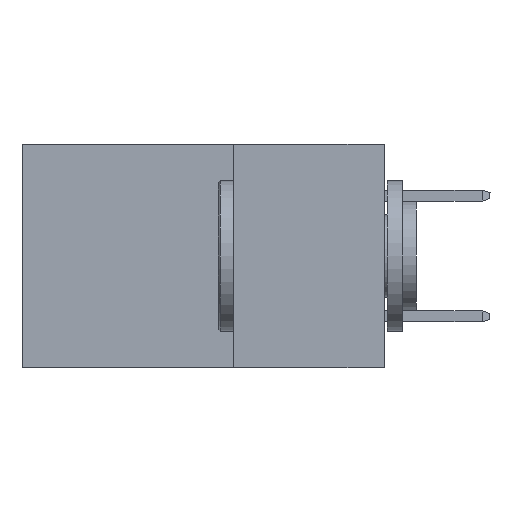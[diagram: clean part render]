
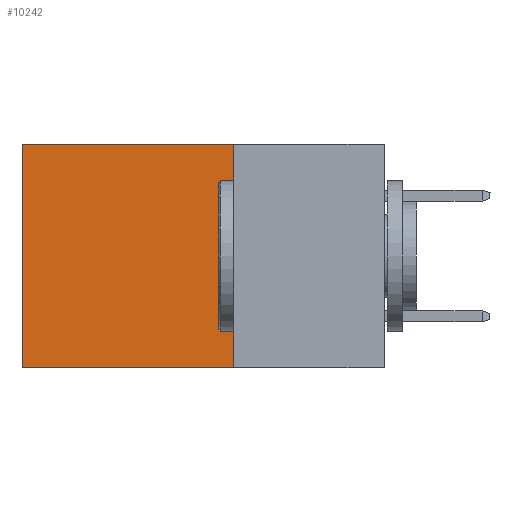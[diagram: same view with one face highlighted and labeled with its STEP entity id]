
A CAD part, left-side view. The second image highlights one B-rep face of the part: STEP entity #10242.
In plain terms, the highlighted planar face has unit normal (-1, 0, 0).
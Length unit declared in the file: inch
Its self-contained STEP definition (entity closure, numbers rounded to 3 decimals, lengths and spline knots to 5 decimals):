
#322 = ORIENTED_EDGE ( 'NONE', *, *, #11833, .F. ) ;
#599 = PLANE ( 'NONE',  #3656 ) ;
#931 = FACE_OUTER_BOUND ( 'NONE', #4082, .T. ) ;
#969 = VECTOR ( 'NONE', #11041, 39.37008 ) ;
#1170 = LINE ( 'NONE', #14396, #7731 ) ;
#1259 = DIRECTION ( 'NONE',  ( 0., 0., -1. ) ) ;
#1739 = LINE ( 'NONE', #15676, #4783 ) ;
#1925 = DIRECTION ( 'NONE',  ( 1., 0., 0. ) ) ;
#2004 = CARTESIAN_POINT ( 'NONE',  ( 0.298, 0.25, -0.37 ) ) ;
#3013 = LINE ( 'NONE', #5563, #969 ) ;
#3249 = DIRECTION ( 'NONE',  ( 0., 0., -1. ) ) ;
#3656 = AXIS2_PLACEMENT_3D ( 'NONE', #16466, #1925, #3249 ) ;
#4034 = CARTESIAN_POINT ( 'NONE',  ( 0.298, 0.25, 0. ) ) ;
#4082 = EDGE_LOOP ( 'NONE', ( #4154, #11042, #322, #10776 ) ) ;
#4154 = ORIENTED_EDGE ( 'NONE', *, *, #12080, .T. ) ;
#4472 = EDGE_CURVE ( 'NONE', #7704, #12834, #1739, .T. ) ;
#4566 = VECTOR ( 'NONE', #14187, 39.37008 ) ;
#4781 = CARTESIAN_POINT ( 'NONE',  ( 0.298, 0.25, -0.37 ) ) ;
#4783 = VECTOR ( 'NONE', #7977, 39.37008 ) ;
#5176 = EDGE_CURVE ( 'NONE', #15212, #11227, #9521, .T. ) ;
#5563 = CARTESIAN_POINT ( 'NONE',  ( 0.298, 0.6, 0. ) ) ;
#7704 = VERTEX_POINT ( 'NONE', #4034 ) ;
#7731 = VECTOR ( 'NONE', #1259, 39.37008 ) ;
#7977 = DIRECTION ( 'NONE',  ( 0., 1., 0. ) ) ;
#9449 = CARTESIAN_POINT ( 'NONE',  ( 0.298, 0.6, -0.37 ) ) ;
#9521 = LINE ( 'NONE', #4781, #4566 ) ;
#10242 = ADVANCED_FACE ( 'NONE', ( #931 ), #599, .F. ) ;
#10776 = ORIENTED_EDGE ( 'NONE', *, *, #4472, .T. ) ;
#11041 = DIRECTION ( 'NONE',  ( 0., 0., -1. ) ) ;
#11042 = ORIENTED_EDGE ( 'NONE', *, *, #5176, .F. ) ;
#11227 = VERTEX_POINT ( 'NONE', #9449 ) ;
#11833 = EDGE_CURVE ( 'NONE', #7704, #15212, #1170, .T. ) ;
#12080 = EDGE_CURVE ( 'NONE', #12834, #11227, #3013, .T. ) ;
#12834 = VERTEX_POINT ( 'NONE', #16276 ) ;
#14187 = DIRECTION ( 'NONE',  ( 0., 1., 0. ) ) ;
#14396 = CARTESIAN_POINT ( 'NONE',  ( 0.298, 0.25, 0. ) ) ;
#15212 = VERTEX_POINT ( 'NONE', #2004 ) ;
#15676 = CARTESIAN_POINT ( 'NONE',  ( 0.298, 0.25, 0. ) ) ;
#16276 = CARTESIAN_POINT ( 'NONE',  ( 0.298, 0.6, 0. ) ) ;
#16466 = CARTESIAN_POINT ( 'NONE',  ( 0.298, 0.25, 0. ) ) ;
